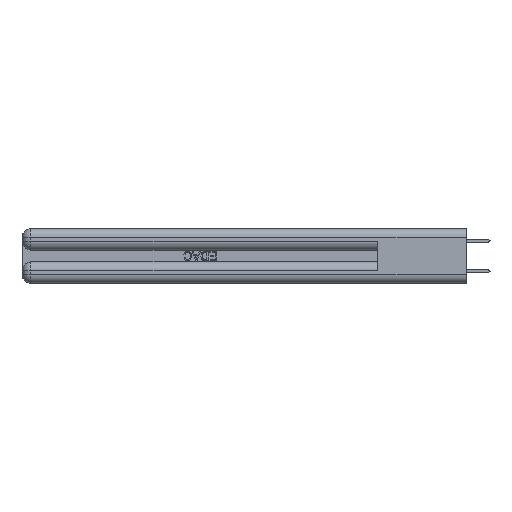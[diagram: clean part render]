
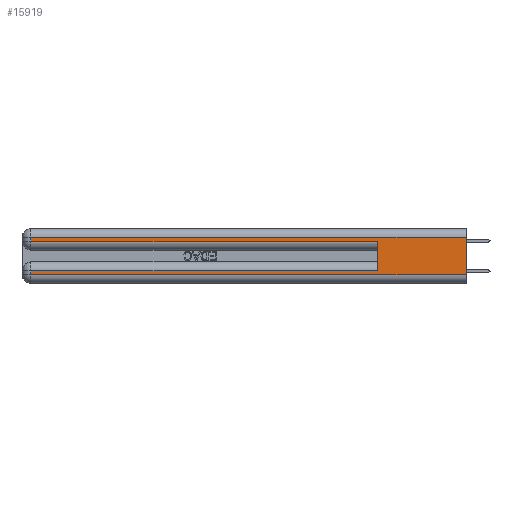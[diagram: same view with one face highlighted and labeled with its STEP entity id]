
A CAD part, left-side view. The second image highlights one B-rep face of the part: STEP entity #15919.
In plain terms, the highlighted planar face has unit normal (-1, 0, 0).
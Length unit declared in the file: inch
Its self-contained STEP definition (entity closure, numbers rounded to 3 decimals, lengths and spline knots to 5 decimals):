
#13 = EDGE_CURVE ( 'NONE', #6600, #17880, #3927, .T. ) ;
#130 = EDGE_CURVE ( 'NONE', #6297, #22005, #24540, .T. ) ;
#1025 = ORIENTED_EDGE ( 'NONE', *, *, #23258, .F. ) ;
#3927 = LINE ( 'NONE', #36231, #38199 ) ;
#4327 = VECTOR ( 'NONE', #12701, 39.37008 ) ;
#4585 = VECTOR ( 'NONE', #46893, 39.37008 ) ;
#4893 = CARTESIAN_POINT ( 'NONE',  ( 0., 0., 0.31 ) ) ;
#4941 = VERTEX_POINT ( 'NONE', #34809 ) ;
#6297 = VERTEX_POINT ( 'NONE', #8977 ) ;
#6600 = VERTEX_POINT ( 'NONE', #42439 ) ;
#7292 = CARTESIAN_POINT ( 'NONE',  ( 0., 0.6, 0.145 ) ) ;
#7683 = CARTESIAN_POINT ( 'NONE',  ( 0., 2.94, 0.06 ) ) ;
#8805 = EDGE_CURVE ( 'NONE', #15527, #6600, #33051, .T. ) ;
#8977 = CARTESIAN_POINT ( 'NONE',  ( 0., 2.94, 0.085 ) ) ;
#9434 = ORIENTED_EDGE ( 'NONE', *, *, #23677, .T. ) ;
#10003 = CARTESIAN_POINT ( 'NONE',  ( 0., 0.6, 0.285 ) ) ;
#10177 = CARTESIAN_POINT ( 'NONE',  ( 0., 2.94, 0.31 ) ) ;
#10364 = ORIENTED_EDGE ( 'NONE', *, *, #27725, .T. ) ;
#11594 = VECTOR ( 'NONE', #29056, 39.37008 ) ;
#12701 = DIRECTION ( 'NONE',  ( 0., -1., 0. ) ) ;
#13065 = VECTOR ( 'NONE', #37616, 39.37008 ) ;
#13305 = EDGE_LOOP ( 'NONE', ( #1025, #36526, #34899, #38670, #22173, #9434, #19517, #10364 ) ) ;
#13312 = EDGE_CURVE ( 'NONE', #19978, #15527, #25052, .T. ) ;
#15527 = VERTEX_POINT ( 'NONE', #10177 ) ;
#15919 = ADVANCED_FACE ( 'NONE', ( #43076 ), #46031, .F. ) ;
#17385 = DIRECTION ( 'NONE',  ( 0., 0., -1. ) ) ;
#17880 = VERTEX_POINT ( 'NONE', #10003 ) ;
#18492 = CARTESIAN_POINT ( 'NONE',  ( 0., 0., 0.37 ) ) ;
#18613 = DIRECTION ( 'NONE',  ( 0., 0., -1. ) ) ;
#19330 = VECTOR ( 'NONE', #18613, 39.37008 ) ;
#19517 = ORIENTED_EDGE ( 'NONE', *, *, #130, .T. ) ;
#19978 = VERTEX_POINT ( 'NONE', #31225 ) ;
#21760 = EDGE_CURVE ( 'NONE', #29704, #17880, #29886, .T. ) ;
#22005 = VERTEX_POINT ( 'NONE', #7683 ) ;
#22173 = ORIENTED_EDGE ( 'NONE', *, *, #21760, .F. ) ;
#22270 = DIRECTION ( 'NONE',  ( 0., 1., 0. ) ) ;
#23258 = EDGE_CURVE ( 'NONE', #19978, #4941, #25201, .T. ) ;
#23380 = AXIS2_PLACEMENT_3D ( 'NONE', #42510, #46178, #35468 ) ;
#23391 = CARTESIAN_POINT ( 'NONE',  ( 0., 0., 0.06 ) ) ;
#23677 = EDGE_CURVE ( 'NONE', #29704, #6297, #40001, .T. ) ;
#24540 = LINE ( 'NONE', #29813, #19330 ) ;
#25052 = LINE ( 'NONE', #4893, #13065 ) ;
#25201 = LINE ( 'NONE', #18492, #4585 ) ;
#27725 = EDGE_CURVE ( 'NONE', #22005, #4941, #37448, .T. ) ;
#28901 = CARTESIAN_POINT ( 'NONE',  ( 0., 0., 0.085 ) ) ;
#29056 = DIRECTION ( 'NONE',  ( 0., 0., 1. ) ) ;
#29161 = VECTOR ( 'NONE', #22270, 39.37008 ) ;
#29704 = VERTEX_POINT ( 'NONE', #32642 ) ;
#29813 = CARTESIAN_POINT ( 'NONE',  ( 0., 2.94, 0.37 ) ) ;
#29886 = LINE ( 'NONE', #7292, #11594 ) ;
#31225 = CARTESIAN_POINT ( 'NONE',  ( 0., 0., 0.31 ) ) ;
#32395 = CARTESIAN_POINT ( 'NONE',  ( 0., 2.94, 0.37 ) ) ;
#32574 = DIRECTION ( 'NONE',  ( 0., -1., 0. ) ) ;
#32642 = CARTESIAN_POINT ( 'NONE',  ( 0., 0.6, 0.085 ) ) ;
#33051 = LINE ( 'NONE', #32395, #39907 ) ;
#34809 = CARTESIAN_POINT ( 'NONE',  ( 0., 0., 0.06 ) ) ;
#34899 = ORIENTED_EDGE ( 'NONE', *, *, #8805, .T. ) ;
#35468 = DIRECTION ( 'NONE',  ( 0., 0., -1. ) ) ;
#36231 = CARTESIAN_POINT ( 'NONE',  ( 0., 0., 0.285 ) ) ;
#36526 = ORIENTED_EDGE ( 'NONE', *, *, #13312, .T. ) ;
#37448 = LINE ( 'NONE', #23391, #4327 ) ;
#37616 = DIRECTION ( 'NONE',  ( 0., 1., 0. ) ) ;
#38199 = VECTOR ( 'NONE', #32574, 39.37008 ) ;
#38670 = ORIENTED_EDGE ( 'NONE', *, *, #13, .T. ) ;
#39907 = VECTOR ( 'NONE', #17385, 39.37008 ) ;
#40001 = LINE ( 'NONE', #28901, #29161 ) ;
#42439 = CARTESIAN_POINT ( 'NONE',  ( 0., 2.94, 0.285 ) ) ;
#42510 = CARTESIAN_POINT ( 'NONE',  ( 0., 0., 0.37 ) ) ;
#43076 = FACE_OUTER_BOUND ( 'NONE', #13305, .T. ) ;
#46031 = PLANE ( 'NONE',  #23380 ) ;
#46178 = DIRECTION ( 'NONE',  ( 1., 0., 0. ) ) ;
#46893 = DIRECTION ( 'NONE',  ( 0., 0., -1. ) ) ;
